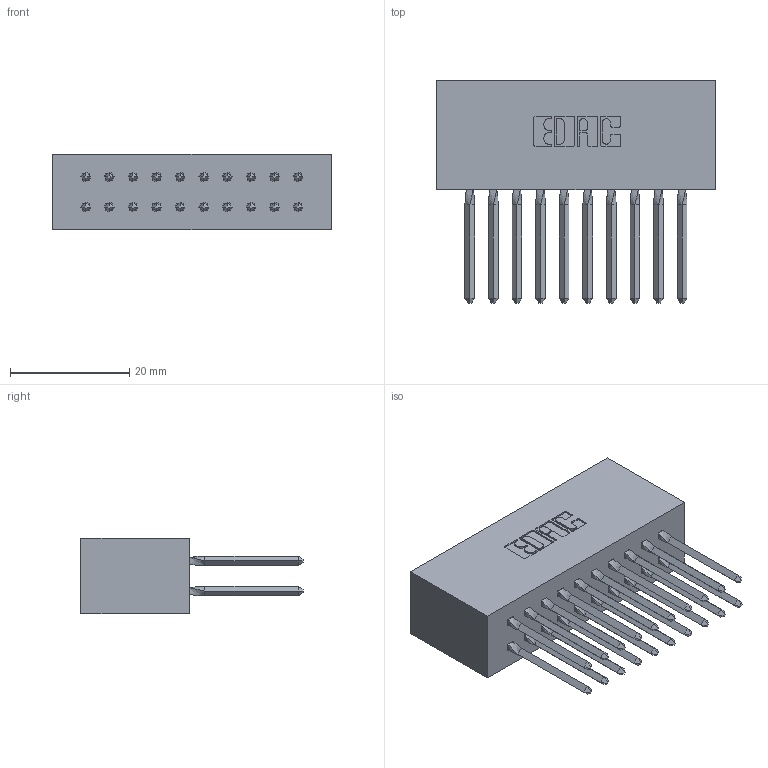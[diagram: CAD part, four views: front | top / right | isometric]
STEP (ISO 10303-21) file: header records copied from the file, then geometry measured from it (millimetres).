
FILE_DESCRIPTION (( 'STEP AP203' ), '1' );
FILE_NAME ('317-020-542-801.STEP', '2020-02-27T16:44:51', ( '' ), ( '' ), 'SwSTEP 2.0', 'SolidWorks 2016', '' );
FILE_SCHEMA (( 'CONFIG_CONTROL_DESIGN' ));
Length unit declared in the file: inch
Products named in the file (3): 317-020-542-801; 317-290-003_542; 317 Part_Lugless
Assembly tree (21 placements, depth 2):
  317-020-542-801
    317 Part_Lugless
    317-290-003_542  x20
Bounding box: 46.84 x 37.34 x 12.7 mm (x, y, z)
Volume: 8388.5 mm3; surface area: 10814.9 mm2
Topology: 21 solids, 21 shells, 1230 faces, 3439 edges, 2198 vertices
Faces by surface type: plane 970, cylinder 180, bspline 80
Entity records: 17527 total; most frequent: CARTESIAN_POINT 3301, ORIENTED_EDGE 2964, DIRECTION 2542, EDGE_CURVE 1482, LINE 1320, VECTOR 1320, VERTEX_POINT 982, AXIS2_PLACEMENT_3D 611
